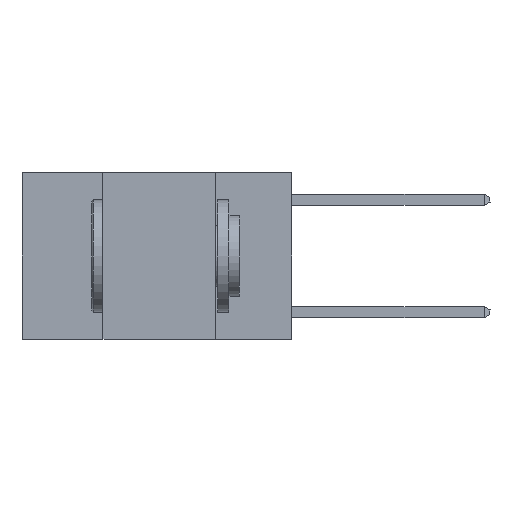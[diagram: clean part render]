
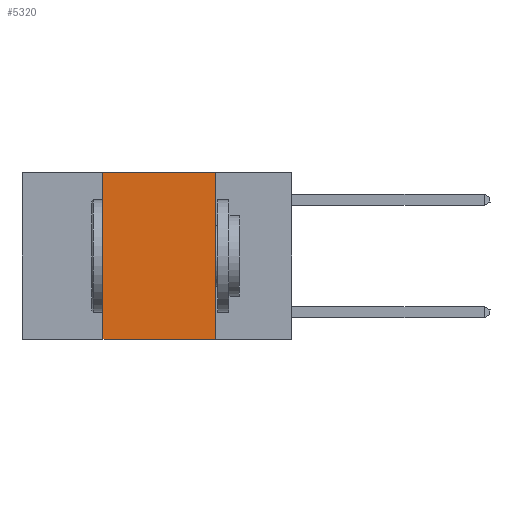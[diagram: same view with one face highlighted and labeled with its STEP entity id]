
A CAD part, left-side view. The second image highlights one B-rep face of the part: STEP entity #5320.
In plain terms, the highlighted planar face has unit normal (-1, 0, 0).
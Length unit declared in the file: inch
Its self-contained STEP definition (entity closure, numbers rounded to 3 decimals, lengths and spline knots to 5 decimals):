
#1751 = EDGE_CURVE ( 'NONE', #27228, #13506, #29853, .T. ) ;
#1826 = DIRECTION ( 'NONE',  ( 0., 0., -1. ) ) ;
#2374 = VECTOR ( 'NONE', #20074, 39.37008 ) ;
#2878 = VERTEX_POINT ( 'NONE', #18466 ) ;
#5320 = ADVANCED_FACE ( 'NONE', ( #24926 ), #7543, .F. ) ;
#6213 = VECTOR ( 'NONE', #8989, 39.37008 ) ;
#6615 = ORIENTED_EDGE ( 'NONE', *, *, #16536, .T. ) ;
#7364 = ORIENTED_EDGE ( 'NONE', *, *, #8452, .F. ) ;
#7543 = PLANE ( 'NONE',  #17908 ) ;
#8452 = EDGE_CURVE ( 'NONE', #13506, #2878, #21777, .T. ) ;
#8989 = DIRECTION ( 'NONE',  ( 0., -1., 0. ) ) ;
#9488 = EDGE_LOOP ( 'NONE', ( #11811, #7364, #29572, #6615 ) ) ;
#10879 = EDGE_CURVE ( 'NONE', #2878, #29545, #24276, .T. ) ;
#11811 = ORIENTED_EDGE ( 'NONE', *, *, #10879, .F. ) ;
#12390 = CARTESIAN_POINT ( 'NONE',  ( 0., 0.17, -0.37 ) ) ;
#13506 = VERTEX_POINT ( 'NONE', #32036 ) ;
#14457 = CARTESIAN_POINT ( 'NONE',  ( 0., 0.17, 0. ) ) ;
#14460 = DIRECTION ( 'NONE',  ( 0., -1., 0. ) ) ;
#14768 = CARTESIAN_POINT ( 'NONE',  ( 0., 0.42, -0.37 ) ) ;
#14827 = CARTESIAN_POINT ( 'NONE',  ( 0., 0.42, 0. ) ) ;
#16536 = EDGE_CURVE ( 'NONE', #27228, #29545, #17747, .T. ) ;
#17577 = CARTESIAN_POINT ( 'NONE',  ( 0., 0.6, 0. ) ) ;
#17586 = CARTESIAN_POINT ( 'NONE',  ( 0., 0.6, -0.37 ) ) ;
#17747 = LINE ( 'NONE', #17586, #19106 ) ;
#17908 = AXIS2_PLACEMENT_3D ( 'NONE', #17577, #27533, #22639 ) ;
#18466 = CARTESIAN_POINT ( 'NONE',  ( 0., 0.17, 0. ) ) ;
#19106 = VECTOR ( 'NONE', #14460, 39.37008 ) ;
#20074 = DIRECTION ( 'NONE',  ( 0., 0., 1. ) ) ;
#21619 = CARTESIAN_POINT ( 'NONE',  ( 0., 0.6, 0. ) ) ;
#21777 = LINE ( 'NONE', #21619, #6213 ) ;
#22639 = DIRECTION ( 'NONE',  ( 0., 0., -1. ) ) ;
#23007 = VECTOR ( 'NONE', #1826, 39.37008 ) ;
#24276 = LINE ( 'NONE', #14457, #23007 ) ;
#24926 = FACE_OUTER_BOUND ( 'NONE', #9488, .T. ) ;
#27228 = VERTEX_POINT ( 'NONE', #14768 ) ;
#27533 = DIRECTION ( 'NONE',  ( 1., 0., 0. ) ) ;
#29545 = VERTEX_POINT ( 'NONE', #12390 ) ;
#29572 = ORIENTED_EDGE ( 'NONE', *, *, #1751, .F. ) ;
#29853 = LINE ( 'NONE', #14827, #2374 ) ;
#32036 = CARTESIAN_POINT ( 'NONE',  ( 0., 0.42, 0. ) ) ;
